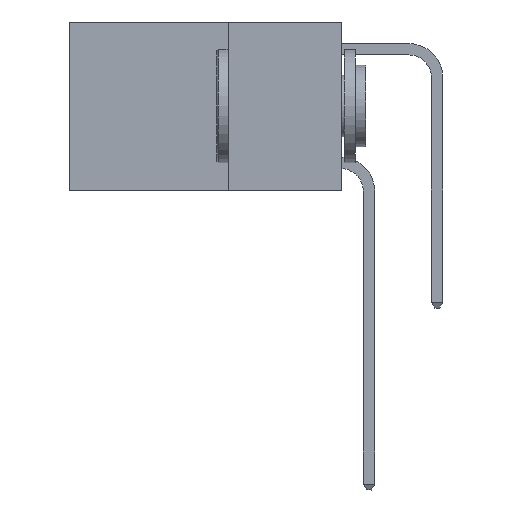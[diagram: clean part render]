
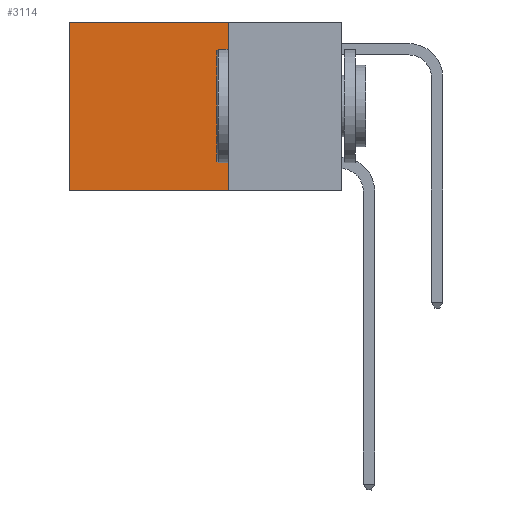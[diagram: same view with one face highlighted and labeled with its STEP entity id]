
A CAD part, left-side view. The second image highlights one B-rep face of the part: STEP entity #3114.
In plain terms, the highlighted planar face has unit normal (-1, 0, 0).
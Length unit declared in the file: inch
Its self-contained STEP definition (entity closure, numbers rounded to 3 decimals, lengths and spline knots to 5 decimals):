
#40 = DIRECTION ( 'NONE',  ( 0., 0., -1. ) ) ;
#180 = CARTESIAN_POINT ( 'NONE',  ( 0.2625, 0.25, -0.37 ) ) ;
#183 = VECTOR ( 'NONE', #10215, 39.37008 ) ;
#420 = VERTEX_POINT ( 'NONE', #180 ) ;
#1071 = DIRECTION ( 'NONE',  ( 1., 0., 0. ) ) ;
#1579 = DIRECTION ( 'NONE',  ( 0., 0., -1. ) ) ;
#1983 = EDGE_LOOP ( 'NONE', ( #8586, #8905, #8106, #9169 ) ) ;
#2322 = DIRECTION ( 'NONE',  ( 0., 1., 0. ) ) ;
#2670 = VERTEX_POINT ( 'NONE', #4754 ) ;
#3016 = LINE ( 'NONE', #8121, #183 ) ;
#3114 = ADVANCED_FACE ( 'NONE', ( #9585 ), #7499, .F. ) ;
#3254 = VECTOR ( 'NONE', #1579, 39.37008 ) ;
#3339 = CARTESIAN_POINT ( 'NONE',  ( 0.2625, 0.25, -0.37 ) ) ;
#4579 = EDGE_CURVE ( 'NONE', #420, #8849, #10520, .T. ) ;
#4667 = AXIS2_PLACEMENT_3D ( 'NONE', #10622, #1071, #40 ) ;
#4754 = CARTESIAN_POINT ( 'NONE',  ( 0.2625, 0.25, 0. ) ) ;
#5453 = CARTESIAN_POINT ( 'NONE',  ( 0.2625, 0.6, 0. ) ) ;
#6119 = EDGE_CURVE ( 'NONE', #6922, #8849, #11131, .T. ) ;
#6922 = VERTEX_POINT ( 'NONE', #5453 ) ;
#7499 = PLANE ( 'NONE',  #4667 ) ;
#7576 = LINE ( 'NONE', #10755, #12199 ) ;
#7930 = CARTESIAN_POINT ( 'NONE',  ( 0.2625, 0.6, 0. ) ) ;
#8106 = ORIENTED_EDGE ( 'NONE', *, *, #9930, .F. ) ;
#8121 = CARTESIAN_POINT ( 'NONE',  ( 0.2625, 0.25, 0. ) ) ;
#8390 = CARTESIAN_POINT ( 'NONE',  ( 0.2625, 0.6, -0.37 ) ) ;
#8586 = ORIENTED_EDGE ( 'NONE', *, *, #6119, .T. ) ;
#8849 = VERTEX_POINT ( 'NONE', #8390 ) ;
#8905 = ORIENTED_EDGE ( 'NONE', *, *, #4579, .F. ) ;
#9169 = ORIENTED_EDGE ( 'NONE', *, *, #10043, .T. ) ;
#9585 = FACE_OUTER_BOUND ( 'NONE', #1983, .T. ) ;
#9613 = DIRECTION ( 'NONE',  ( 0., 1., 0. ) ) ;
#9930 = EDGE_CURVE ( 'NONE', #2670, #420, #3016, .T. ) ;
#10043 = EDGE_CURVE ( 'NONE', #2670, #6922, #7576, .T. ) ;
#10215 = DIRECTION ( 'NONE',  ( 0., 0., -1. ) ) ;
#10520 = LINE ( 'NONE', #3339, #12679 ) ;
#10622 = CARTESIAN_POINT ( 'NONE',  ( 0.2625, 0.25, 0. ) ) ;
#10755 = CARTESIAN_POINT ( 'NONE',  ( 0.2625, 0.25, 0. ) ) ;
#11131 = LINE ( 'NONE', #7930, #3254 ) ;
#12199 = VECTOR ( 'NONE', #2322, 39.37008 ) ;
#12679 = VECTOR ( 'NONE', #9613, 39.37008 ) ;
